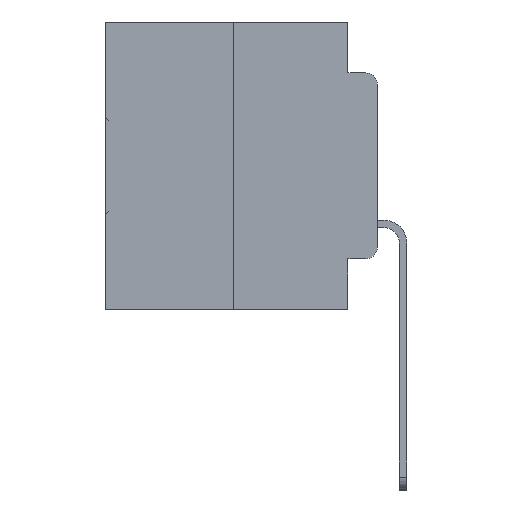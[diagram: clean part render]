
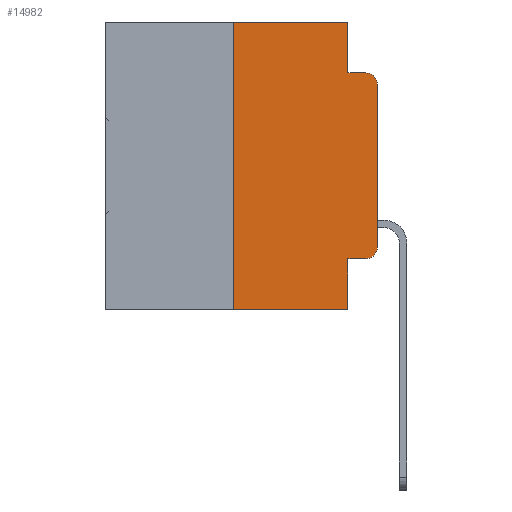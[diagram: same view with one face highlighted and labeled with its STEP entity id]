
A CAD part, left-side view. The second image highlights one B-rep face of the part: STEP entity #14982.
In plain terms, the highlighted planar face has unit normal (-1, 0, 0).
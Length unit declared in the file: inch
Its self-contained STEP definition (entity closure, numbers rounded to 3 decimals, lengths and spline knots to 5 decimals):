
#2259 = DIRECTION ( 'NONE',  ( 0., -1., 0. ) ) ;
#2880 = VECTOR ( 'NONE', #13546, 39.37008 ) ;
#3401 = EDGE_CURVE ( 'NONE', #9875, #13679, #11354, .T. ) ;
#3410 = VECTOR ( 'NONE', #20769, 39.37008 ) ;
#3590 = DIRECTION ( 'NONE',  ( -1., 0., 0. ) ) ;
#3739 = VERTEX_POINT ( 'NONE', #9907 ) ;
#3878 = CIRCLE ( 'NONE', #12671, 0.02 ) ;
#4196 = VERTEX_POINT ( 'NONE', #28917 ) ;
#5222 = PLANE ( 'NONE',  #24395 ) ;
#5237 = EDGE_CURVE ( 'NONE', #14368, #3739, #19977, .T. ) ;
#6183 = VECTOR ( 'NONE', #13400, 39.37008 ) ;
#6299 = VECTOR ( 'NONE', #15371, 39.37008 ) ;
#6833 = VERTEX_POINT ( 'NONE', #11767 ) ;
#7932 = FACE_OUTER_BOUND ( 'NONE', #10199, .T. ) ;
#7963 = CARTESIAN_POINT ( 'NONE',  ( 0., 0.051, 0. ) ) ;
#7986 = DIRECTION ( 'NONE',  ( 1., 0., 0. ) ) ;
#8140 = CARTESIAN_POINT ( 'NONE',  ( 0., 0., -0.3915 ) ) ;
#8776 = LINE ( 'NONE', #7963, #21504 ) ;
#9875 = VERTEX_POINT ( 'NONE', #21296 ) ;
#9907 = CARTESIAN_POINT ( 'NONE',  ( 0., 0.25, 0. ) ) ;
#10175 = LINE ( 'NONE', #23454, #2880 ) ;
#10199 = EDGE_LOOP ( 'NONE', ( #11119, #11572, #20645, #17885, #25934, #12403, #30849, #25961, #14792, #19550 ) ) ;
#10628 = CARTESIAN_POINT ( 'NONE',  ( 0., 0.051, -0.0885 ) ) ;
#10695 = LINE ( 'NONE', #10628, #3410 ) ;
#10849 = CARTESIAN_POINT ( 'NONE',  ( 0., 0.051, 0. ) ) ;
#10851 = CARTESIAN_POINT ( 'NONE',  ( 0., 0.25, 0. ) ) ;
#10855 = VERTEX_POINT ( 'NONE', #8140 ) ;
#11119 = ORIENTED_EDGE ( 'NONE', *, *, #28969, .T. ) ;
#11270 = VERTEX_POINT ( 'NONE', #32644 ) ;
#11354 = LINE ( 'NONE', #10849, #29504 ) ;
#11572 = ORIENTED_EDGE ( 'NONE', *, *, #27368, .T. ) ;
#11744 = CARTESIAN_POINT ( 'NONE',  ( 0., 0.051, -0.5 ) ) ;
#11767 = CARTESIAN_POINT ( 'NONE',  ( 0., 0.051, 0. ) ) ;
#11851 = LINE ( 'NONE', #15149, #19362 ) ;
#12403 = ORIENTED_EDGE ( 'NONE', *, *, #5237, .F. ) ;
#12564 = LINE ( 'NONE', #32357, #6299 ) ;
#12671 = AXIS2_PLACEMENT_3D ( 'NONE', #19280, #3590, #21740 ) ;
#12900 = CARTESIAN_POINT ( 'NONE',  ( 0., 0.02, -0.1085 ) ) ;
#12904 = AXIS2_PLACEMENT_3D ( 'NONE', #12900, #30096, #15420 ) ;
#13397 = DIRECTION ( 'NONE',  ( 0., 0., -1. ) ) ;
#13400 = DIRECTION ( 'NONE',  ( 0., 0., 1. ) ) ;
#13546 = DIRECTION ( 'NONE',  ( 0., -1., 0. ) ) ;
#13679 = VERTEX_POINT ( 'NONE', #11744 ) ;
#14137 = EDGE_CURVE ( 'NONE', #6833, #20159, #8776, .T. ) ;
#14368 = VERTEX_POINT ( 'NONE', #22015 ) ;
#14792 = ORIENTED_EDGE ( 'NONE', *, *, #32763, .T. ) ;
#14982 = ADVANCED_FACE ( 'NONE', ( #7932 ), #5222, .F. ) ;
#15149 = CARTESIAN_POINT ( 'NONE',  ( 0., 0.051, -0.4115 ) ) ;
#15371 = DIRECTION ( 'NONE',  ( 0., 0., 1. ) ) ;
#15420 = DIRECTION ( 'NONE',  ( 0., 0., -1. ) ) ;
#15692 = VECTOR ( 'NONE', #2259, 39.37008 ) ;
#16092 = CARTESIAN_POINT ( 'NONE',  ( 0., 0.051, -0.0885 ) ) ;
#16343 = VERTEX_POINT ( 'NONE', #19428 ) ;
#17885 = ORIENTED_EDGE ( 'NONE', *, *, #14137, .F. ) ;
#19216 = EDGE_CURVE ( 'NONE', #20159, #11270, #10695, .T. ) ;
#19280 = CARTESIAN_POINT ( 'NONE',  ( 0., 0.02, -0.3915 ) ) ;
#19362 = VECTOR ( 'NONE', #29861, 39.37008 ) ;
#19428 = CARTESIAN_POINT ( 'NONE',  ( 0., 0., -0.1085 ) ) ;
#19550 = ORIENTED_EDGE ( 'NONE', *, *, #24742, .T. ) ;
#19977 = LINE ( 'NONE', #10851, #6183 ) ;
#20159 = VERTEX_POINT ( 'NONE', #16092 ) ;
#20645 = ORIENTED_EDGE ( 'NONE', *, *, #19216, .F. ) ;
#20739 = DIRECTION ( 'NONE',  ( 0., 0., -1. ) ) ;
#20769 = DIRECTION ( 'NONE',  ( 0., -1., 0. ) ) ;
#21296 = CARTESIAN_POINT ( 'NONE',  ( 0., 0.051, -0.4115 ) ) ;
#21504 = VECTOR ( 'NONE', #20739, 39.37008 ) ;
#21740 = DIRECTION ( 'NONE',  ( 0., 0., -1. ) ) ;
#21752 = EDGE_CURVE ( 'NONE', #3739, #6833, #22336, .T. ) ;
#22015 = CARTESIAN_POINT ( 'NONE',  ( 0., 0.25, -0.5 ) ) ;
#22336 = LINE ( 'NONE', #32592, #15692 ) ;
#23194 = CARTESIAN_POINT ( 'NONE',  ( 0., 0.473, 0. ) ) ;
#23454 = CARTESIAN_POINT ( 'NONE',  ( 0., 0.473, -0.5 ) ) ;
#24395 = AXIS2_PLACEMENT_3D ( 'NONE', #23194, #7986, #25608 ) ;
#24742 = EDGE_CURVE ( 'NONE', #4196, #10855, #3878, .T. ) ;
#25608 = DIRECTION ( 'NONE',  ( 0., 0., -1. ) ) ;
#25934 = ORIENTED_EDGE ( 'NONE', *, *, #21752, .F. ) ;
#25961 = ORIENTED_EDGE ( 'NONE', *, *, #3401, .F. ) ;
#26114 = CIRCLE ( 'NONE', #12904, 0.02 ) ;
#27368 = EDGE_CURVE ( 'NONE', #16343, #11270, #26114, .T. ) ;
#27572 = EDGE_CURVE ( 'NONE', #14368, #13679, #10175, .T. ) ;
#28917 = CARTESIAN_POINT ( 'NONE',  ( 0., 0.02, -0.4115 ) ) ;
#28969 = EDGE_CURVE ( 'NONE', #10855, #16343, #12564, .T. ) ;
#29504 = VECTOR ( 'NONE', #13397, 39.37008 ) ;
#29861 = DIRECTION ( 'NONE',  ( 0., -1., 0. ) ) ;
#30096 = DIRECTION ( 'NONE',  ( -1., 0., 0. ) ) ;
#30849 = ORIENTED_EDGE ( 'NONE', *, *, #27572, .T. ) ;
#32357 = CARTESIAN_POINT ( 'NONE',  ( 0., 0., 0. ) ) ;
#32592 = CARTESIAN_POINT ( 'NONE',  ( 0., 0.473, 0. ) ) ;
#32644 = CARTESIAN_POINT ( 'NONE',  ( 0., 0.02, -0.0885 ) ) ;
#32763 = EDGE_CURVE ( 'NONE', #9875, #4196, #11851, .T. ) ;
